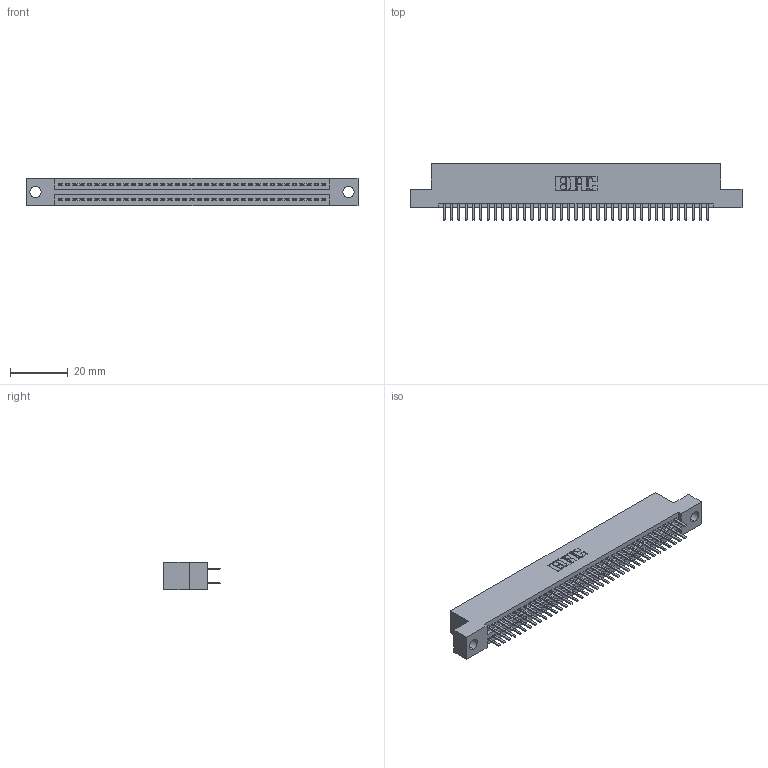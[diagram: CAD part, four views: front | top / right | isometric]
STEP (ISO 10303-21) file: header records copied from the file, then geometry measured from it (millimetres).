
FILE_DESCRIPTION (( 'STEP AP203' ), '1' );
FILE_NAME ('345-074-520-204.STEP', '2018-10-02T11:02:23', ( '' ), ( '' ), 'SwSTEP 2.0', 'SolidWorks 2016', '' );
FILE_SCHEMA (( 'CONFIG_CONTROL_DESIGN' ));
Length unit declared in the file: inch
Products named in the file (3): 345-074-520-204; 345 Part_Flush Mounting Lugs - 0.156 Dia-TH; 345-292-001_345-293-120
Assembly tree (75 placements, depth 2):
  345-074-520-204
    345 Part_Flush Mounting Lugs - 0.156 Dia-TH
    345-292-001_345-293-120  x74
Bounding box: 115.19 x 19.68 x 9.4 mm (x, y, z)
Volume: 11022.8 mm3; surface area: 15942.7 mm2
Topology: 75 solids, 75 shells, 4122 faces, 11959 edges, 7774 vertices
Faces by surface type: plane 2670, cylinder 1452
Entity records: 29821 total; most frequent: CARTESIAN_POINT 5016, ORIENTED_EDGE 4938, DIRECTION 4417, EDGE_CURVE 2469, VECTOR 2185, LINE 2185, VERTEX_POINT 1642, AXIS2_PLACEMENT_3D 1116
